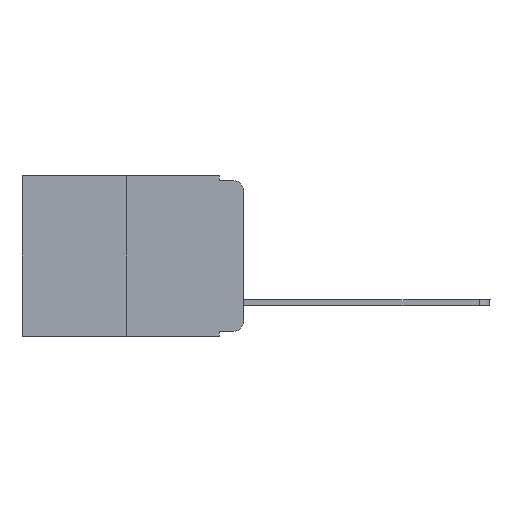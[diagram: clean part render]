
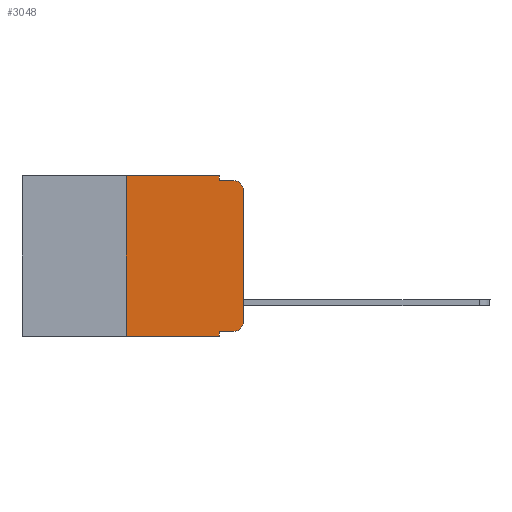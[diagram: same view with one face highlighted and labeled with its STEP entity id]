
A CAD part, left-side view. The second image highlights one B-rep face of the part: STEP entity #3048.
In plain terms, the highlighted planar face has unit normal (-1, 0, 0).
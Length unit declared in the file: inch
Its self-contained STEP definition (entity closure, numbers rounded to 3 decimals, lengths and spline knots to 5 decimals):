
#101 = LINE ( 'NONE', #11638, #13946 ) ;
#141 = CARTESIAN_POINT ( 'NONE',  ( 0., 0., -0.313 ) ) ;
#293 = DIRECTION ( 'NONE',  ( -1., 0., 0. ) ) ;
#1160 = AXIS2_PLACEMENT_3D ( 'NONE', #16642, #1580, #8600 ) ;
#1392 = DIRECTION ( 'NONE',  ( 0., 0., 1. ) ) ;
#1580 = DIRECTION ( 'NONE',  ( 1., 0., 0. ) ) ;
#1913 = VERTEX_POINT ( 'NONE', #10985 ) ;
#2016 = CIRCLE ( 'NONE', #8007, 0.02 ) ;
#2171 = EDGE_CURVE ( 'NONE', #6837, #2903, #12155, .T. ) ;
#2272 = LINE ( 'NONE', #6006, #21088 ) ;
#2697 = CARTESIAN_POINT ( 'NONE',  ( 0., 0.02, -0.03 ) ) ;
#2903 = VERTEX_POINT ( 'NONE', #13226 ) ;
#3048 = ADVANCED_FACE ( 'NONE', ( #9932 ), #3557, .F. ) ;
#3207 = CARTESIAN_POINT ( 'NONE',  ( 0., 0.25, -0.343 ) ) ;
#3557 = PLANE ( 'NONE',  #1160 ) ;
#3569 = VERTEX_POINT ( 'NONE', #11171 ) ;
#3597 = CARTESIAN_POINT ( 'NONE',  ( 0., 0.051, 0. ) ) ;
#4032 = VECTOR ( 'NONE', #17108, 39.37008 ) ;
#4599 = VERTEX_POINT ( 'NONE', #3207 ) ;
#4782 = LINE ( 'NONE', #14566, #5269 ) ;
#4806 = CARTESIAN_POINT ( 'NONE',  ( 0., 0., 0. ) ) ;
#5176 = EDGE_CURVE ( 'NONE', #3569, #20350, #18524, .T. ) ;
#5269 = VECTOR ( 'NONE', #11255, 39.37008 ) ;
#5557 = CARTESIAN_POINT ( 'NONE',  ( 0., 0.051, -0.343 ) ) ;
#5753 = ORIENTED_EDGE ( 'NONE', *, *, #9777, .F. ) ;
#6002 = AXIS2_PLACEMENT_3D ( 'NONE', #2697, #12794, #9388 ) ;
#6006 = CARTESIAN_POINT ( 'NONE',  ( 0., 0.473, -0.343 ) ) ;
#6107 = ORIENTED_EDGE ( 'NONE', *, *, #2171, .T. ) ;
#6160 = VECTOR ( 'NONE', #20584, 39.37008 ) ;
#6312 = CARTESIAN_POINT ( 'NONE',  ( 0., 0.051, -0.333 ) ) ;
#6837 = VERTEX_POINT ( 'NONE', #6312 ) ;
#8007 = AXIS2_PLACEMENT_3D ( 'NONE', #13606, #293, #20322 ) ;
#8075 = VERTEX_POINT ( 'NONE', #16088 ) ;
#8230 = ORIENTED_EDGE ( 'NONE', *, *, #16248, .F. ) ;
#8359 = ORIENTED_EDGE ( 'NONE', *, *, #18556, .F. ) ;
#8372 = ORIENTED_EDGE ( 'NONE', *, *, #16192, .T. ) ;
#8390 = VECTOR ( 'NONE', #18136, 39.37008 ) ;
#8600 = DIRECTION ( 'NONE',  ( 0., 0., -1. ) ) ;
#8620 = ORIENTED_EDGE ( 'NONE', *, *, #12355, .T. ) ;
#8690 = CARTESIAN_POINT ( 'NONE',  ( 0., 0.051, -0.01 ) ) ;
#9163 = ORIENTED_EDGE ( 'NONE', *, *, #10555, .T. ) ;
#9388 = DIRECTION ( 'NONE',  ( 0., 0., -1. ) ) ;
#9777 = EDGE_CURVE ( 'NONE', #20350, #13996, #21109, .T. ) ;
#9932 = FACE_OUTER_BOUND ( 'NONE', #17965, .T. ) ;
#10555 = EDGE_CURVE ( 'NONE', #13743, #8075, #17994, .T. ) ;
#10831 = DIRECTION ( 'NONE',  ( 0., -1., 0. ) ) ;
#10985 = CARTESIAN_POINT ( 'NONE',  ( 0., 0.25, 0. ) ) ;
#11171 = CARTESIAN_POINT ( 'NONE',  ( 0., 0.051, 0. ) ) ;
#11255 = DIRECTION ( 'NONE',  ( 0., 0., 1. ) ) ;
#11425 = CARTESIAN_POINT ( 'NONE',  ( 0., 0.051, -0.01 ) ) ;
#11638 = CARTESIAN_POINT ( 'NONE',  ( 0., 0.473, 0. ) ) ;
#12140 = VERTEX_POINT ( 'NONE', #5557 ) ;
#12155 = LINE ( 'NONE', #16903, #4032 ) ;
#12355 = EDGE_CURVE ( 'NONE', #8075, #13996, #20024, .T. ) ;
#12794 = DIRECTION ( 'NONE',  ( -1., 0., 0. ) ) ;
#12856 = VECTOR ( 'NONE', #18963, 39.37008 ) ;
#13161 = CARTESIAN_POINT ( 'NONE',  ( 0., 0.051, 0. ) ) ;
#13226 = CARTESIAN_POINT ( 'NONE',  ( 0., 0.02, -0.333 ) ) ;
#13355 = VECTOR ( 'NONE', #1392, 39.37008 ) ;
#13405 = DIRECTION ( 'NONE',  ( 0., -1., 0. ) ) ;
#13606 = CARTESIAN_POINT ( 'NONE',  ( 0., 0.02, -0.313 ) ) ;
#13743 = VERTEX_POINT ( 'NONE', #141 ) ;
#13946 = VECTOR ( 'NONE', #13405, 39.37008 ) ;
#13996 = VERTEX_POINT ( 'NONE', #14771 ) ;
#14566 = CARTESIAN_POINT ( 'NONE',  ( 0., 0.25, 0. ) ) ;
#14771 = CARTESIAN_POINT ( 'NONE',  ( 0., 0.02, -0.01 ) ) ;
#15278 = ORIENTED_EDGE ( 'NONE', *, *, #5176, .F. ) ;
#15359 = EDGE_CURVE ( 'NONE', #6837, #12140, #21606, .T. ) ;
#16088 = CARTESIAN_POINT ( 'NONE',  ( 0., 0., -0.03 ) ) ;
#16192 = EDGE_CURVE ( 'NONE', #2903, #13743, #2016, .T. ) ;
#16248 = EDGE_CURVE ( 'NONE', #1913, #3569, #101, .T. ) ;
#16642 = CARTESIAN_POINT ( 'NONE',  ( 0., 0.473, 0. ) ) ;
#16903 = CARTESIAN_POINT ( 'NONE',  ( 0., 0.051, -0.333 ) ) ;
#17108 = DIRECTION ( 'NONE',  ( 0., -1., 0. ) ) ;
#17655 = ORIENTED_EDGE ( 'NONE', *, *, #19667, .T. ) ;
#17965 = EDGE_LOOP ( 'NONE', ( #9163, #8620, #5753, #15278, #8230, #8359, #17655, #20912, #6107, #8372 ) ) ;
#17994 = LINE ( 'NONE', #4806, #13355 ) ;
#18136 = DIRECTION ( 'NONE',  ( 0., -1., 0. ) ) ;
#18524 = LINE ( 'NONE', #3597, #12856 ) ;
#18556 = EDGE_CURVE ( 'NONE', #4599, #1913, #4782, .T. ) ;
#18963 = DIRECTION ( 'NONE',  ( 0., 0., -1. ) ) ;
#19667 = EDGE_CURVE ( 'NONE', #4599, #12140, #2272, .T. ) ;
#20024 = CIRCLE ( 'NONE', #6002, 0.02 ) ;
#20322 = DIRECTION ( 'NONE',  ( 0., 0., -1. ) ) ;
#20350 = VERTEX_POINT ( 'NONE', #8690 ) ;
#20584 = DIRECTION ( 'NONE',  ( 0., 0., -1. ) ) ;
#20912 = ORIENTED_EDGE ( 'NONE', *, *, #15359, .F. ) ;
#21088 = VECTOR ( 'NONE', #10831, 39.37008 ) ;
#21109 = LINE ( 'NONE', #11425, #8390 ) ;
#21606 = LINE ( 'NONE', #13161, #6160 ) ;
